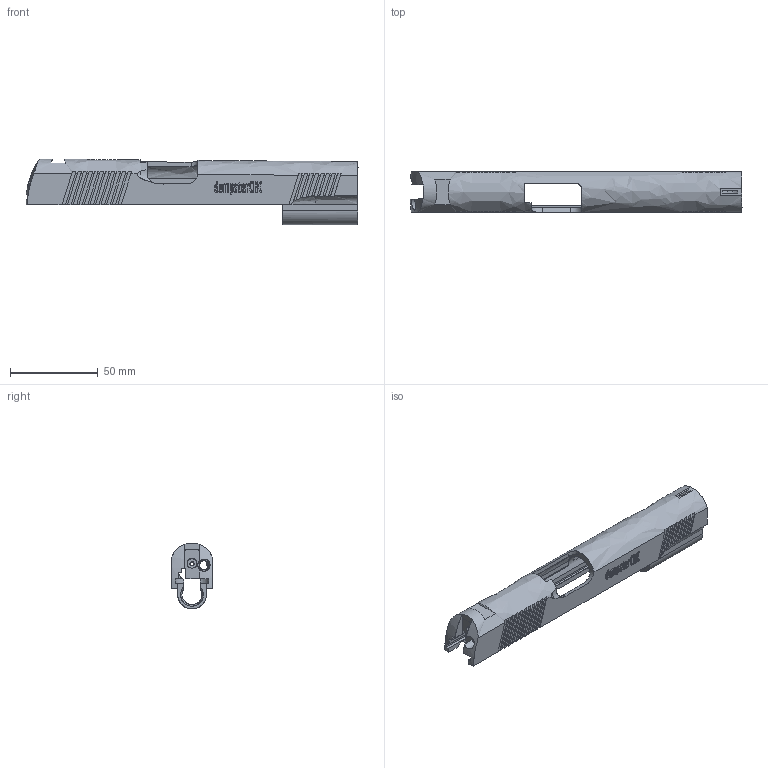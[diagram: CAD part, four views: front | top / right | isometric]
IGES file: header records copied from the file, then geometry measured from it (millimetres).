
Global section: file name: 1911 Slide Model.igs; native system: Virtual 7.7.6 NLO; preprocessor: Exchange 1.0; author: Tim Winkfein; organization: dumpsterCNC; date: 060412.004653; units: inch
Bounding box: 189.36 x 23.24 x 37.55 mm (x, y, z)
Surface area: 29586 mm2 (no closed solid volume)
Topology: 0 solids, 0 shells, 1189 faces, 7257 edges, 7257 vertices
Faces by surface type: bspline 1189
